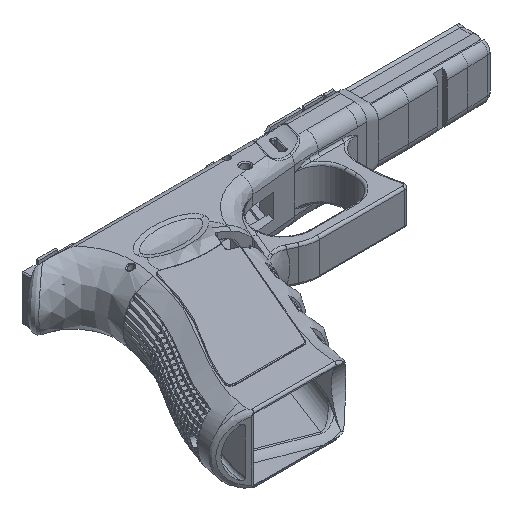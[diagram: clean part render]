
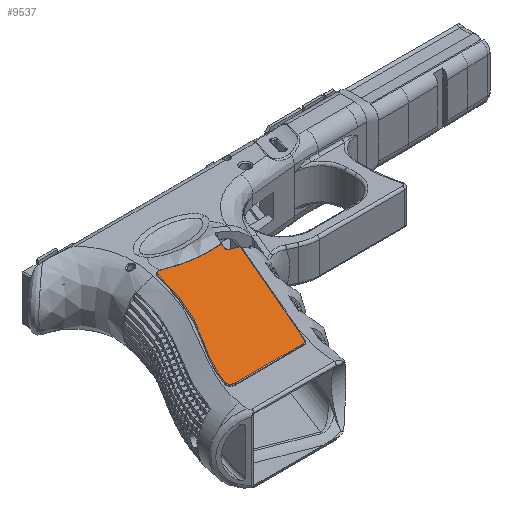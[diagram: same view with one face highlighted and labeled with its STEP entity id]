
A CAD part, isometric view. The second image highlights one B-rep face of the part: STEP entity #9537.
In plain terms, the highlighted planar face has unit normal (0, 0, 1).
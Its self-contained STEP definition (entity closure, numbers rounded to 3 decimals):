
#737 = ORIENTED_EDGE ( 'NONE', *, *, #69887, .F. ) ;
#2088 = AXIS2_PLACEMENT_3D ( 'NONE', #85311, #31998, #94306 ) ;
#3943 = EDGE_CURVE ( 'NONE', #42292, #19918, #89970, .T. ) ;
#6473 = CARTESIAN_POINT ( 'NONE',  ( 54.41, 63.593, 14.941 ) ) ;
#7952 = VERTEX_POINT ( 'NONE', #106981 ) ;
#8450 = CARTESIAN_POINT ( 'NONE',  ( 36.884, 14.537, 14.941 ) ) ;
#9537 = ADVANCED_FACE ( 'NONE', ( #35392 ), #43707, .F. ) ;
#10233 = VERTEX_POINT ( 'NONE', #94612 ) ;
#10627 = VERTEX_POINT ( 'NONE', #36884 ) ;
#11181 = CARTESIAN_POINT ( 'NONE',  ( 6.194, 13.462, 14.941 ) ) ;
#14506 = AXIS2_PLACEMENT_3D ( 'NONE', #89926, #36606, #98911 ) ;
#15079 = DIRECTION ( 'NONE',  ( 0., 0., -1. ) ) ;
#15106 = CARTESIAN_POINT ( 'NONE',  ( 32.235, 70.631, 14.941 ) ) ;
#16636 = DIRECTION ( 'NONE',  ( 0., 0., -1. ) ) ;
#18700 = VERTEX_POINT ( 'NONE', #32755 ) ;
#18815 = CARTESIAN_POINT ( 'NONE',  ( 53.595, 64.779, 14.941 ) ) ;
#19918 = VERTEX_POINT ( 'NONE', #15106 ) ;
#21784 = CARTESIAN_POINT ( 'NONE',  ( 29.811, 69.397, 14.941 ) ) ;
#23760 = ORIENTED_EDGE ( 'NONE', *, *, #66472, .T. ) ;
#26209 = DIRECTION ( 'NONE',  ( 0., 0., -1. ) ) ;
#26748 = EDGE_CURVE ( 'NONE', #85644, #101786, #104848, .T. ) ;
#27048 = LINE ( 'NONE', #93667, #95356 ) ;
#27289 = VERTEX_POINT ( 'NONE', #11181 ) ;
#28207 = VECTOR ( 'NONE', #42889, 1000. ) ;
#31576 = AXIS2_PLACEMENT_3D ( 'NONE', #103913, #50502, #112866 ) ;
#31998 = DIRECTION ( 'NONE',  ( 0., 0., -1. ) ) ;
#32755 = CARTESIAN_POINT ( 'NONE',  ( 4.534, 15.875, 14.941 ) ) ;
#33078 = CIRCLE ( 'NONE', #31576, 1.778 ) ;
#35211 = ORIENTED_EDGE ( 'NONE', *, *, #3943, .F. ) ;
#35335 = ORIENTED_EDGE ( 'NONE', *, *, #26748, .T. ) ;
#35392 = FACE_OUTER_BOUND ( 'NONE', #80936, .T. ) ;
#36606 = DIRECTION ( 'NONE',  ( 0., 0., -1. ) ) ;
#36884 = CARTESIAN_POINT ( 'NONE',  ( 54.494, 67.354, 14.941 ) ) ;
#38440 = CIRCLE ( 'NONE', #14506, 86.316 ) ;
#39843 = AXIS2_PLACEMENT_3D ( 'NONE', #42574, #104918, #51490 ) ;
#40398 = CARTESIAN_POINT ( 'NONE',  ( 31.543, 68.994, 14.941 ) ) ;
#42292 = VERTEX_POINT ( 'NONE', #21784 ) ;
#42574 = CARTESIAN_POINT ( 'NONE',  ( 49.685, 111.919, 14.941 ) ) ;
#42889 = DIRECTION ( 'NONE',  ( 0.358, 0.934, 0. ) ) ;
#43707 = PLANE ( 'NONE',  #95398 ) ;
#44207 = CIRCLE ( 'NONE', #87489, 102.555 ) ;
#44617 = ORIENTED_EDGE ( 'NONE', *, *, #108800, .F. ) ;
#45570 = CARTESIAN_POINT ( 'NONE',  ( -70.075, 92.642, 14.941 ) ) ;
#45646 = AXIS2_PLACEMENT_3D ( 'NONE', #69890, #16636, #78892 ) ;
#48191 = EDGE_CURVE ( 'NONE', #10233, #85204, #101352, .T. ) ;
#49211 = DIRECTION ( 'NONE',  ( -1., 0., 0. ) ) ;
#49317 = DIRECTION ( 'NONE',  ( 1., 0., 0. ) ) ;
#49673 = CARTESIAN_POINT ( 'NONE',  ( 54.41, 63.593, 14.941 ) ) ;
#50502 = DIRECTION ( 'NONE',  ( 0., 0., -1. ) ) ;
#50561 = CIRCLE ( 'NONE', #39843, 44.823 ) ;
#51490 = DIRECTION ( 'NONE',  ( 1., 0., 0. ) ) ;
#51716 = CIRCLE ( 'NONE', #73125, 1.778 ) ;
#52583 = CIRCLE ( 'NONE', #45646, 1.27 ) ;
#53637 = ORIENTED_EDGE ( 'NONE', *, *, #76387, .F. ) ;
#54514 = DIRECTION ( 'NONE',  ( 1., 0., 0. ) ) ;
#54821 = VECTOR ( 'NONE', #81905, 1000. ) ;
#62256 = VECTOR ( 'NONE', #106186, 1000. ) ;
#65021 = ORIENTED_EDGE ( 'NONE', *, *, #93635, .T. ) ;
#66192 = CARTESIAN_POINT ( 'NONE',  ( 35.251, 13.462, 14.941 ) ) ;
#66472 = EDGE_CURVE ( 'NONE', #101786, #89479, #52583, .T. ) ;
#66685 = EDGE_CURVE ( 'NONE', #7952, #42292, #44207, .T. ) ;
#67156 = EDGE_CURVE ( 'NONE', #27289, #18700, #33078, .T. ) ;
#68354 = CARTESIAN_POINT ( 'NONE',  ( 35.251, 15.24, 14.941 ) ) ;
#69887 = EDGE_CURVE ( 'NONE', #18700, #7952, #38440, .T. ) ;
#69890 = CARTESIAN_POINT ( 'NONE',  ( 54.865, 64.779, 14.941 ) ) ;
#70323 = CARTESIAN_POINT ( 'NONE',  ( 53.68, 65.234, 14.941 ) ) ;
#71481 = ORIENTED_EDGE ( 'NONE', *, *, #81206, .F. ) ;
#72359 = VERTEX_POINT ( 'NONE', #66192 ) ;
#73125 = AXIS2_PLACEMENT_3D ( 'NONE', #68354, #15079, #77331 ) ;
#76387 = EDGE_CURVE ( 'NONE', #72359, #27289, #27048, .T. ) ;
#76880 = EDGE_CURVE ( 'NONE', #10233, #85644, #102288, .T. ) ;
#77331 = DIRECTION ( 'NONE',  ( 1., 0., 0. ) ) ;
#78892 = DIRECTION ( 'NONE',  ( -1., 0., 0. ) ) ;
#79529 = CARTESIAN_POINT ( 'NONE',  ( 85.161, -14.94, 14.941 ) ) ;
#80936 = EDGE_LOOP ( 'NONE', ( #92281, #84692, #35335, #23760, #65021, #44617, #35211, #114255, #737, #96835, #53637, #71481 ) ) ;
#81206 = EDGE_CURVE ( 'NONE', #85204, #72359, #51716, .T. ) ;
#81905 = DIRECTION ( 'NONE',  ( -0.934, 0.358, 0. ) ) ;
#84393 = CARTESIAN_POINT ( 'NONE',  ( 36.884, 14.537, 14.941 ) ) ;
#84692 = ORIENTED_EDGE ( 'NONE', *, *, #76880, .T. ) ;
#85204 = VERTEX_POINT ( 'NONE', #84393 ) ;
#85311 = CARTESIAN_POINT ( 'NONE',  ( 54.865, 64.779, 14.941 ) ) ;
#85644 = VERTEX_POINT ( 'NONE', #49673 ) ;
#87489 = AXIS2_PLACEMENT_3D ( 'NONE', #45570, #107942, #54514 ) ;
#88488 = DIRECTION ( 'NONE',  ( 1., 0., 0. ) ) ;
#89479 = VERTEX_POINT ( 'NONE', #70323 ) ;
#89926 = CARTESIAN_POINT ( 'NONE',  ( 85.161, -14.94, 14.941 ) ) ;
#89970 = CIRCLE ( 'NONE', #105650, 1.778 ) ;
#92281 = ORIENTED_EDGE ( 'NONE', *, *, #48191, .F. ) ;
#93635 = EDGE_CURVE ( 'NONE', #89479, #10627, #93723, .T. ) ;
#93667 = CARTESIAN_POINT ( 'NONE',  ( 6.194, 13.462, 14.941 ) ) ;
#93723 = LINE ( 'NONE', #96252, #28207 ) ;
#94306 = DIRECTION ( 'NONE',  ( -1., 0., 0. ) ) ;
#94612 = CARTESIAN_POINT ( 'NONE',  ( 57.5, 62.407, 14.941 ) ) ;
#95356 = VECTOR ( 'NONE', #49211, 1000. ) ;
#95398 = AXIS2_PLACEMENT_3D ( 'NONE', #79529, #26209, #88488 ) ;
#96252 = CARTESIAN_POINT ( 'NONE',  ( 54.541, 67.477, 14.941 ) ) ;
#96835 = ORIENTED_EDGE ( 'NONE', *, *, #67156, .F. ) ;
#98911 = DIRECTION ( 'NONE',  ( 1., 0., 0. ) ) ;
#101352 = LINE ( 'NONE', #8450, #62256 ) ;
#101786 = VERTEX_POINT ( 'NONE', #18815 ) ;
#102288 = LINE ( 'NONE', #6473, #54821 ) ;
#102733 = DIRECTION ( 'NONE',  ( 0., 0., -1. ) ) ;
#103913 = CARTESIAN_POINT ( 'NONE',  ( 6.194, 15.24, 14.941 ) ) ;
#104848 = CIRCLE ( 'NONE', #2088, 1.27 ) ;
#104918 = DIRECTION ( 'NONE',  ( 0., 0., 1. ) ) ;
#105650 = AXIS2_PLACEMENT_3D ( 'NONE', #40398, #102733, #49317 ) ;
#106186 = DIRECTION ( 'NONE',  ( -0.396, -0.918, 0. ) ) ;
#106981 = CARTESIAN_POINT ( 'NONE',  ( 14.217, 34.226, 14.941 ) ) ;
#107942 = DIRECTION ( 'NONE',  ( 0., 0., 1. ) ) ;
#108800 = EDGE_CURVE ( 'NONE', #19918, #10627, #50561, .T. ) ;
#112866 = DIRECTION ( 'NONE',  ( 1., 0., 0. ) ) ;
#114255 = ORIENTED_EDGE ( 'NONE', *, *, #66685, .F. ) ;
